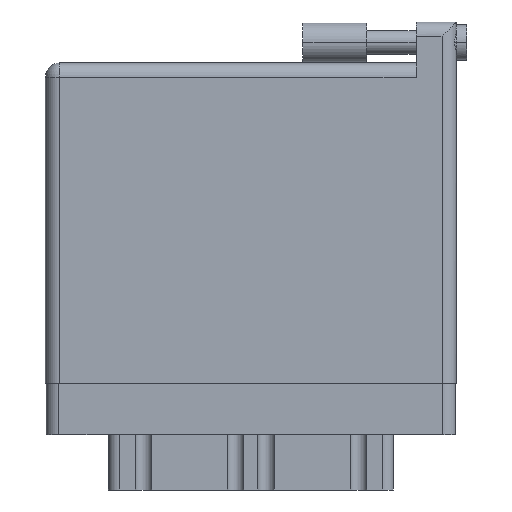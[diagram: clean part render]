
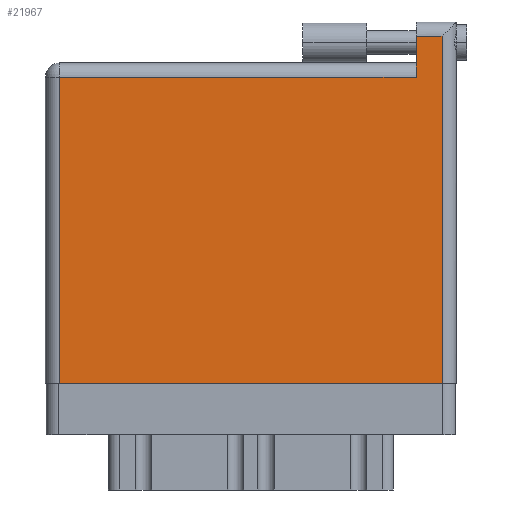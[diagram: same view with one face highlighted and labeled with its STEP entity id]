
A CAD part, front view. The second image highlights one B-rep face of the part: STEP entity #21967.
In plain terms, the highlighted face is planar.
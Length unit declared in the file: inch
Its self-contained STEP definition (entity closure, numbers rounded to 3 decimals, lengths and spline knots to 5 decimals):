
#1434 = EDGE_CURVE ( 'NONE', #10370, #9466, #27820, .T. ) ;
#2118 = CARTESIAN_POINT ( 'NONE',  ( 0., 0., 0. ) ) ;
#2954 = CARTESIAN_POINT ( 'NONE',  ( 0.07, 1.496, 0. ) ) ;
#4191 = CARTESIAN_POINT ( 'NONE',  ( 0., 1.496, 0. ) ) ;
#4595 = ORIENTED_EDGE ( 'NONE', *, *, #14396, .T. ) ;
#4604 = VECTOR ( 'NONE', #11200, 39.37008 ) ;
#4714 = VECTOR ( 'NONE', #21932, 39.37008 ) ;
#4942 = CARTESIAN_POINT ( 'NONE',  ( 1.811, 1.696, 0. ) ) ;
#5802 = CARTESIAN_POINT ( 'NONE',  ( 1.938, 1.696, 0. ) ) ;
#7917 = FACE_OUTER_BOUND ( 'NONE', #9389, .T. ) ;
#8217 = VERTEX_POINT ( 'NONE', #5802 ) ;
#8464 = LINE ( 'NONE', #14131, #4604 ) ;
#9319 = ORIENTED_EDGE ( 'NONE', *, *, #35775, .T. ) ;
#9389 = EDGE_LOOP ( 'NONE', ( #17685, #34403, #9319, #4595, #21726, #27998 ) ) ;
#9466 = VERTEX_POINT ( 'NONE', #10536 ) ;
#9600 = EDGE_CURVE ( 'NONE', #28577, #10370, #22298, .T. ) ;
#10370 = VERTEX_POINT ( 'NONE', #2954 ) ;
#10536 = CARTESIAN_POINT ( 'NONE',  ( 0.07, 0., 0. ) ) ;
#11200 = DIRECTION ( 'NONE',  ( -1., 0., 0. ) ) ;
#11247 = VERTEX_POINT ( 'NONE', #35201 ) ;
#13299 = VECTOR ( 'NONE', #33456, 39.37008 ) ;
#13474 = VECTOR ( 'NONE', #28005, 39.37008 ) ;
#13629 = VECTOR ( 'NONE', #18394, 39.37008 ) ;
#14131 = CARTESIAN_POINT ( 'NONE',  ( 0., 1.696, 0. ) ) ;
#14396 = EDGE_CURVE ( 'NONE', #36024, #28577, #27331, .T. ) ;
#17685 = ORIENTED_EDGE ( 'NONE', *, *, #33488, .T. ) ;
#18394 = DIRECTION ( 'NONE',  ( 0., -1., 0. ) ) ;
#21230 = LINE ( 'NONE', #24703, #13299 ) ;
#21726 = ORIENTED_EDGE ( 'NONE', *, *, #9600, .T. ) ;
#21932 = DIRECTION ( 'NONE',  ( -1., 0., 0. ) ) ;
#21967 = ADVANCED_FACE ( 'NONE', ( #7917 ), #38109, .F. ) ;
#22119 = VECTOR ( 'NONE', #37181, 39.37008 ) ;
#22170 = CARTESIAN_POINT ( 'NONE',  ( 0.07, 0., 0. ) ) ;
#22298 = LINE ( 'NONE', #4191, #4714 ) ;
#24703 = CARTESIAN_POINT ( 'NONE',  ( 1.938, 1.766, 0. ) ) ;
#26623 = CARTESIAN_POINT ( 'NONE',  ( 1.811, 1.496, 0. ) ) ;
#27331 = LINE ( 'NONE', #35710, #13629 ) ;
#27820 = LINE ( 'NONE', #22170, #13474 ) ;
#27998 = ORIENTED_EDGE ( 'NONE', *, *, #1434, .T. ) ;
#28005 = DIRECTION ( 'NONE',  ( 0., -1., 0. ) ) ;
#28577 = VERTEX_POINT ( 'NONE', #26623 ) ;
#29153 = DIRECTION ( 'NONE',  ( 0., 0., -1. ) ) ;
#31721 = LINE ( 'NONE', #2118, #22119 ) ;
#32053 = CARTESIAN_POINT ( 'NONE',  ( 0., 1.566, 0. ) ) ;
#32244 = DIRECTION ( 'NONE',  ( -1., 0., 0. ) ) ;
#33456 = DIRECTION ( 'NONE',  ( 0., 1., 0. ) ) ;
#33488 = EDGE_CURVE ( 'NONE', #9466, #11247, #31721, .T. ) ;
#33639 = AXIS2_PLACEMENT_3D ( 'NONE', #32053, #29153, #32244 ) ;
#34403 = ORIENTED_EDGE ( 'NONE', *, *, #35182, .T. ) ;
#35182 = EDGE_CURVE ( 'NONE', #11247, #8217, #21230, .T. ) ;
#35201 = CARTESIAN_POINT ( 'NONE',  ( 1.938, 0., 0. ) ) ;
#35710 = CARTESIAN_POINT ( 'NONE',  ( 1.811, 1.766, 0. ) ) ;
#35775 = EDGE_CURVE ( 'NONE', #8217, #36024, #8464, .T. ) ;
#36024 = VERTEX_POINT ( 'NONE', #4942 ) ;
#37181 = DIRECTION ( 'NONE',  ( 1., 0., 0. ) ) ;
#38109 = PLANE ( 'NONE',  #33639 ) ;
